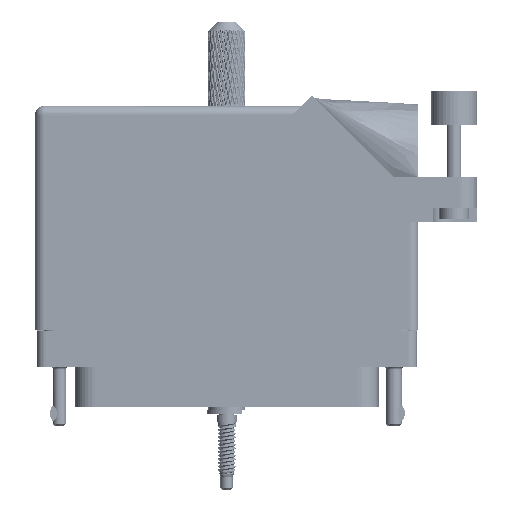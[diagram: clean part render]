
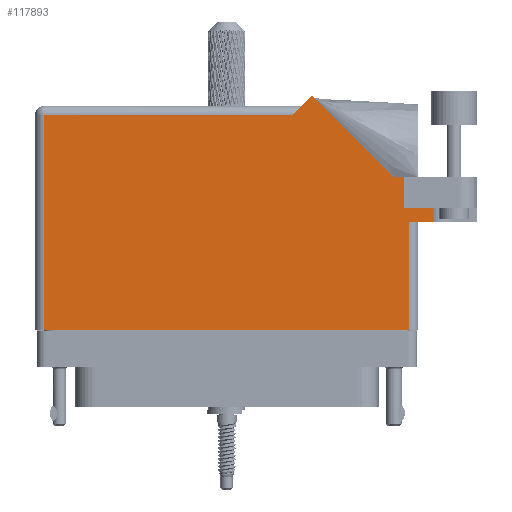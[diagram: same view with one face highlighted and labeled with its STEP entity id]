
A CAD part, front view. The second image highlights one B-rep face of the part: STEP entity #117893.
In plain terms, the highlighted face is planar.
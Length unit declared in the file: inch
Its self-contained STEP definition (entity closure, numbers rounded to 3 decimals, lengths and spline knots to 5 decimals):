
#529 = ORIENTED_EDGE ( 'NONE', *, *, #94820, .T. ) ;
#641 = EDGE_CURVE ( 'NONE', #24491, #61837, #71108, .T. ) ;
#5277 = FACE_OUTER_BOUND ( 'NONE', #6754, .T. ) ;
#5925 = PLANE ( 'NONE',  #110958 ) ;
#6645 = VERTEX_POINT ( 'NONE', #62803 ) ;
#6754 = EDGE_LOOP ( 'NONE', ( #109102, #87650, #59866, #71933, #85854, #69775, #97325, #61392, #87264, #98074, #529 ) ) ;
#7577 = DIRECTION ( 'NONE',  ( -0.707, -0.707, 0. ) ) ;
#7791 = DIRECTION ( 'NONE',  ( -1., 0., 0. ) ) ;
#9744 = EDGE_CURVE ( 'NONE', #10788, #86388, #100869, .T. ) ;
#10788 = VERTEX_POINT ( 'NONE', #28472 ) ;
#11238 = EDGE_CURVE ( 'NONE', #6645, #76897, #45178, .T. ) ;
#13155 = DIRECTION ( 'NONE',  ( -1., 0., 0. ) ) ;
#14050 = DIRECTION ( 'NONE',  ( -0.707, 0.707, 0. ) ) ;
#15139 = CARTESIAN_POINT ( 'NONE',  ( -1.244, -0.1, 0.455 ) ) ;
#18231 = VECTOR ( 'NONE', #13155, 39.37008 ) ;
#19470 = LINE ( 'NONE', #15139, #37957 ) ;
#19754 = DIRECTION ( 'NONE',  ( 0., 1., 0. ) ) ;
#21602 = CARTESIAN_POINT ( 'NONE',  ( 1.244, 0.637, 0.455 ) ) ;
#22132 = CARTESIAN_POINT ( 'NONE',  ( 1.706, 0.944, 0.455 ) ) ;
#24491 = VERTEX_POINT ( 'NONE', #49945 ) ;
#26528 = LINE ( 'NONE', #71163, #29621 ) ;
#27797 = VECTOR ( 'NONE', #105853, 39.37008 ) ;
#28472 = CARTESIAN_POINT ( 'NONE',  ( 1.206, 0.731, 0.455 ) ) ;
#29621 = VECTOR ( 'NONE', #81074, 39.37008 ) ;
#35480 = DIRECTION ( 'NONE',  ( 0., 0., -1. ) ) ;
#36322 = CARTESIAN_POINT ( 'NONE',  ( -1.306, 1.43, 0.455 ) ) ;
#37957 = VECTOR ( 'NONE', #102809, 39.37008 ) ;
#45178 = LINE ( 'NONE', #72957, #80713 ) ;
#49945 = CARTESIAN_POINT ( 'NONE',  ( 1.244, -0.1, 0.455 ) ) ;
#49951 = CARTESIAN_POINT ( 'NONE',  ( 1.4075, 0.731, 0.455 ) ) ;
#58157 = EDGE_CURVE ( 'NONE', #76897, #114040, #92187, .T. ) ;
#59715 = EDGE_CURVE ( 'NONE', #86388, #6645, #99739, .T. ) ;
#59866 = ORIENTED_EDGE ( 'NONE', *, *, #73157, .T. ) ;
#60820 = DIRECTION ( 'NONE',  ( 0., 1., 0. ) ) ;
#61392 = ORIENTED_EDGE ( 'NONE', *, *, #11238, .T. ) ;
#61837 = VERTEX_POINT ( 'NONE', #21602 ) ;
#62652 = CARTESIAN_POINT ( 'NONE',  ( 1.4075, 0.637, 0.455 ) ) ;
#62803 = CARTESIAN_POINT ( 'NONE',  ( 1.14042, 0.944, 0.455 ) ) ;
#63398 = VERTEX_POINT ( 'NONE', #49951 ) ;
#63977 = VERTEX_POINT ( 'NONE', #62652 ) ;
#64652 = LINE ( 'NONE', #102856, #27797 ) ;
#66036 = VECTOR ( 'NONE', #7577, 39.37008 ) ;
#66354 = DIRECTION ( 'NONE',  ( 0., -1., 0. ) ) ;
#67014 = CARTESIAN_POINT ( 'NONE',  ( -1.306, 1.368, 0.455 ) ) ;
#69334 = EDGE_CURVE ( 'NONE', #63398, #63977, #125944, .T. ) ;
#69775 = ORIENTED_EDGE ( 'NONE', *, *, #9744, .T. ) ;
#71108 = LINE ( 'NONE', #78711, #117175 ) ;
#71163 = CARTESIAN_POINT ( 'NONE',  ( 1.206, 0.731, 0.455 ) ) ;
#71933 = ORIENTED_EDGE ( 'NONE', *, *, #69334, .F. ) ;
#72019 = CARTESIAN_POINT ( 'NONE',  ( 0.58371, 1.50071, 0.455 ) ) ;
#72062 = CARTESIAN_POINT ( 'NONE',  ( 1.206, 0.731, 0.455 ) ) ;
#72957 = CARTESIAN_POINT ( 'NONE',  ( 1.14042, 0.944, 0.455 ) ) ;
#73157 = EDGE_CURVE ( 'NONE', #61837, #63977, #100724, .T. ) ;
#74776 = VECTOR ( 'NONE', #60820, 39.37008 ) ;
#76318 = CARTESIAN_POINT ( 'NONE',  ( 0.513, 1.43, 0.455 ) ) ;
#76897 = VERTEX_POINT ( 'NONE', #72019 ) ;
#78711 = CARTESIAN_POINT ( 'NONE',  ( 1.244, 0.637, 0.455 ) ) ;
#79134 = EDGE_CURVE ( 'NONE', #114040, #86059, #100441, .T. ) ;
#80713 = VECTOR ( 'NONE', #14050, 39.37008 ) ;
#81074 = DIRECTION ( 'NONE',  ( 1., 0., 0. ) ) ;
#84117 = DIRECTION ( 'NONE',  ( -1., 0., 0. ) ) ;
#85854 = ORIENTED_EDGE ( 'NONE', *, *, #98370, .F. ) ;
#86059 = VERTEX_POINT ( 'NONE', #98072 ) ;
#86388 = VERTEX_POINT ( 'NONE', #96632 ) ;
#87264 = ORIENTED_EDGE ( 'NONE', *, *, #58157, .T. ) ;
#87650 = ORIENTED_EDGE ( 'NONE', *, *, #641, .T. ) ;
#91488 = CARTESIAN_POINT ( 'NONE',  ( 1.306, 0.637, 0.455 ) ) ;
#92187 = LINE ( 'NONE', #76318, #66036 ) ;
#93098 = VECTOR ( 'NONE', #100937, 39.37008 ) ;
#94820 = EDGE_CURVE ( 'NONE', #86059, #108864, #19470, .T. ) ;
#96632 = CARTESIAN_POINT ( 'NONE',  ( 1.206, 0.944, 0.455 ) ) ;
#97325 = ORIENTED_EDGE ( 'NONE', *, *, #59715, .T. ) ;
#98072 = CARTESIAN_POINT ( 'NONE',  ( -1.244, 1.368, 0.455 ) ) ;
#98074 = ORIENTED_EDGE ( 'NONE', *, *, #79134, .T. ) ;
#98370 = EDGE_CURVE ( 'NONE', #10788, #63398, #26528, .T. ) ;
#99739 = LINE ( 'NONE', #22132, #18231 ) ;
#100441 = LINE ( 'NONE', #67014, #111125 ) ;
#100724 = LINE ( 'NONE', #91488, #93098 ) ;
#100869 = LINE ( 'NONE', #72062, #74776 ) ;
#100937 = DIRECTION ( 'NONE',  ( 1., 0., 0. ) ) ;
#101331 = EDGE_CURVE ( 'NONE', #108864, #24491, #64652, .T. ) ;
#102809 = DIRECTION ( 'NONE',  ( 0., -1., 0. ) ) ;
#102856 = CARTESIAN_POINT ( 'NONE',  ( -1.306, -0.1, 0.455 ) ) ;
#105853 = DIRECTION ( 'NONE',  ( 1., 0., 0. ) ) ;
#105962 = CARTESIAN_POINT ( 'NONE',  ( -1.244, -0.1, 0.455 ) ) ;
#108864 = VERTEX_POINT ( 'NONE', #105962 ) ;
#109102 = ORIENTED_EDGE ( 'NONE', *, *, #101331, .T. ) ;
#110958 = AXIS2_PLACEMENT_3D ( 'NONE', #36322, #35480, #84117 ) ;
#111125 = VECTOR ( 'NONE', #7791, 39.37008 ) ;
#114040 = VERTEX_POINT ( 'NONE', #115243 ) ;
#115243 = CARTESIAN_POINT ( 'NONE',  ( 0.451, 1.368, 0.455 ) ) ;
#116555 = CARTESIAN_POINT ( 'NONE',  ( 1.4075, 1.06177, 0.455 ) ) ;
#117175 = VECTOR ( 'NONE', #19754, 39.37008 ) ;
#117893 = ADVANCED_FACE ( 'NONE', ( #5277 ), #5925, .F. ) ;
#122814 = VECTOR ( 'NONE', #66354, 39.37008 ) ;
#125944 = LINE ( 'NONE', #116555, #122814 ) ;
